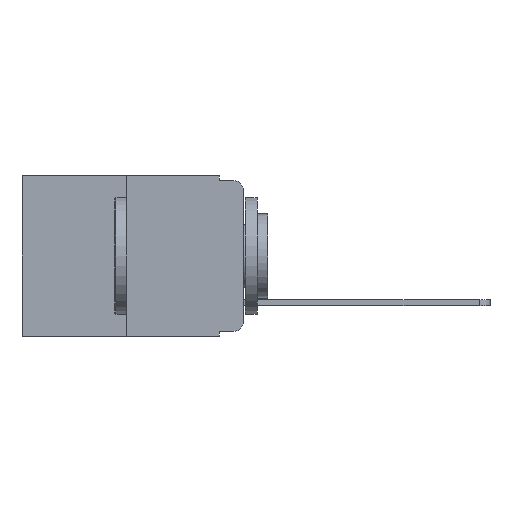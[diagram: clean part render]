
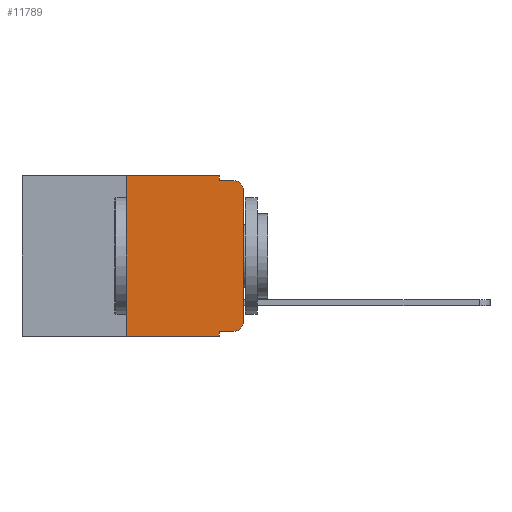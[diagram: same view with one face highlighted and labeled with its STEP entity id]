
A CAD part, left-side view. The second image highlights one B-rep face of the part: STEP entity #11789.
In plain terms, the highlighted planar face has unit normal (-1, 0, 0).
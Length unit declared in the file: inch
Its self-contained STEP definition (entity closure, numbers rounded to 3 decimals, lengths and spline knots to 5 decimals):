
#95 = EDGE_CURVE ( 'NONE', #4473, #4813, #11190, .T. ) ;
#414 = EDGE_CURVE ( 'NONE', #8009, #8805, #6182, .T. ) ;
#613 = EDGE_CURVE ( 'NONE', #2740, #1840, #8915, .T. ) ;
#783 = AXIS2_PLACEMENT_3D ( 'NONE', #10735, #5534, #11582 ) ;
#919 = CARTESIAN_POINT ( 'NONE',  ( 0., 0.051, -0.333 ) ) ;
#976 = LINE ( 'NONE', #11518, #8476 ) ;
#1075 = ORIENTED_EDGE ( 'NONE', *, *, #1500, .T. ) ;
#1089 = DIRECTION ( 'NONE',  ( 0., 0., 1. ) ) ;
#1138 = ORIENTED_EDGE ( 'NONE', *, *, #11715, .T. ) ;
#1239 = ORIENTED_EDGE ( 'NONE', *, *, #414, .F. ) ;
#1320 = ORIENTED_EDGE ( 'NONE', *, *, #1777, .F. ) ;
#1435 = ORIENTED_EDGE ( 'NONE', *, *, #3710, .F. ) ;
#1453 = CARTESIAN_POINT ( 'NONE',  ( 0., 0.02, -0.333 ) ) ;
#1490 = ORIENTED_EDGE ( 'NONE', *, *, #95, .F. ) ;
#1500 = EDGE_CURVE ( 'NONE', #1840, #4595, #9960, .T. ) ;
#1570 = ORIENTED_EDGE ( 'NONE', *, *, #6686, .T. ) ;
#1635 = ORIENTED_EDGE ( 'NONE', *, *, #5709, .F. ) ;
#1747 = CARTESIAN_POINT ( 'NONE',  ( 0., 0.25, 0. ) ) ;
#1765 = ORIENTED_EDGE ( 'NONE', *, *, #7527, .T. ) ;
#1777 = EDGE_CURVE ( 'NONE', #9561, #8009, #2238, .T. ) ;
#1840 = VERTEX_POINT ( 'NONE', #3034 ) ;
#1904 = ORIENTED_EDGE ( 'NONE', *, *, #613, .T. ) ;
#2153 = CARTESIAN_POINT ( 'NONE',  ( 0., 0.051, 0. ) ) ;
#2238 = LINE ( 'NONE', #11919, #7297 ) ;
#2255 = VECTOR ( 'NONE', #10435, 39.37008 ) ;
#2387 = DIRECTION ( 'NONE',  ( 0., 0., -1. ) ) ;
#2417 = DIRECTION ( 'NONE',  ( -1., 0., 0. ) ) ;
#2437 = CARTESIAN_POINT ( 'NONE',  ( 0., 0.02, -0.313 ) ) ;
#2740 = VERTEX_POINT ( 'NONE', #1453 ) ;
#2889 = DIRECTION ( 'NONE',  ( 0., 0., -1. ) ) ;
#3034 = CARTESIAN_POINT ( 'NONE',  ( 0., 0., -0.313 ) ) ;
#3709 = CARTESIAN_POINT ( 'NONE',  ( 0., 0.473, 0. ) ) ;
#3710 = EDGE_CURVE ( 'NONE', #4813, #9561, #11620, .T. ) ;
#4097 = CARTESIAN_POINT ( 'NONE',  ( 0., 0.25, -0.343 ) ) ;
#4186 = CARTESIAN_POINT ( 'NONE',  ( 0., 0., -0.03 ) ) ;
#4473 = VERTEX_POINT ( 'NONE', #4097 ) ;
#4595 = VERTEX_POINT ( 'NONE', #4186 ) ;
#4644 = DIRECTION ( 'NONE',  ( 0., 0., -1. ) ) ;
#4654 = CARTESIAN_POINT ( 'NONE',  ( 0., 0.051, -0.343 ) ) ;
#4674 = DIRECTION ( 'NONE',  ( 0., 0., -1. ) ) ;
#4755 = AXIS2_PLACEMENT_3D ( 'NONE', #3709, #9983, #4674 ) ;
#4813 = VERTEX_POINT ( 'NONE', #1747 ) ;
#4916 = VECTOR ( 'NONE', #8345, 39.37008 ) ;
#5203 = CARTESIAN_POINT ( 'NONE',  ( 0., 0.051, -0.01 ) ) ;
#5318 = CARTESIAN_POINT ( 'NONE',  ( 0., 0.051, -0.01 ) ) ;
#5534 = DIRECTION ( 'NONE',  ( -1., 0., 0. ) ) ;
#5709 = EDGE_CURVE ( 'NONE', #11911, #7623, #10123, .T. ) ;
#5711 = EDGE_LOOP ( 'NONE', ( #1075, #1138, #1239, #1320, #1435, #1490, #1570, #1635, #1765, #1904 ) ) ;
#5879 = CARTESIAN_POINT ( 'NONE',  ( 0., 0., 0. ) ) ;
#6182 = LINE ( 'NONE', #5203, #10528 ) ;
#6450 = CARTESIAN_POINT ( 'NONE',  ( 0., 0.051, 0. ) ) ;
#6574 = CIRCLE ( 'NONE', #783, 0.02 ) ;
#6686 = EDGE_CURVE ( 'NONE', #4473, #7623, #7024, .T. ) ;
#6853 = DIRECTION ( 'NONE',  ( 0., -1., 0. ) ) ;
#6909 = VECTOR ( 'NONE', #1089, 39.37008 ) ;
#7024 = LINE ( 'NONE', #10448, #2255 ) ;
#7231 = CARTESIAN_POINT ( 'NONE',  ( 0., 0.25, 0. ) ) ;
#7248 = DIRECTION ( 'NONE',  ( 0., -1., 0. ) ) ;
#7297 = VECTOR ( 'NONE', #4644, 39.37008 ) ;
#7420 = DIRECTION ( 'NONE',  ( 0., 0., 1. ) ) ;
#7527 = EDGE_CURVE ( 'NONE', #11911, #2740, #976, .T. ) ;
#7597 = CARTESIAN_POINT ( 'NONE',  ( 0., 0.02, -0.01 ) ) ;
#7623 = VERTEX_POINT ( 'NONE', #4654 ) ;
#7656 = AXIS2_PLACEMENT_3D ( 'NONE', #2437, #2417, #2387 ) ;
#7869 = VECTOR ( 'NONE', #2889, 39.37008 ) ;
#8009 = VERTEX_POINT ( 'NONE', #5318 ) ;
#8268 = PLANE ( 'NONE',  #4755 ) ;
#8345 = DIRECTION ( 'NONE',  ( 0., -1., 0. ) ) ;
#8476 = VECTOR ( 'NONE', #7248, 39.37008 ) ;
#8789 = CARTESIAN_POINT ( 'NONE',  ( 0., 0.473, 0. ) ) ;
#8805 = VERTEX_POINT ( 'NONE', #7597 ) ;
#8915 = CIRCLE ( 'NONE', #7656, 0.02 ) ;
#9561 = VERTEX_POINT ( 'NONE', #2153 ) ;
#9800 = FACE_OUTER_BOUND ( 'NONE', #5711, .T. ) ;
#9960 = LINE ( 'NONE', #5879, #11418 ) ;
#9983 = DIRECTION ( 'NONE',  ( 1., 0., 0. ) ) ;
#10123 = LINE ( 'NONE', #6450, #7869 ) ;
#10435 = DIRECTION ( 'NONE',  ( 0., -1., 0. ) ) ;
#10448 = CARTESIAN_POINT ( 'NONE',  ( 0., 0.473, -0.343 ) ) ;
#10528 = VECTOR ( 'NONE', #6853, 39.37008 ) ;
#10735 = CARTESIAN_POINT ( 'NONE',  ( 0., 0.02, -0.03 ) ) ;
#11190 = LINE ( 'NONE', #7231, #6909 ) ;
#11418 = VECTOR ( 'NONE', #7420, 39.37008 ) ;
#11518 = CARTESIAN_POINT ( 'NONE',  ( 0., 0.051, -0.333 ) ) ;
#11582 = DIRECTION ( 'NONE',  ( 0., 0., -1. ) ) ;
#11620 = LINE ( 'NONE', #8789, #4916 ) ;
#11715 = EDGE_CURVE ( 'NONE', #4595, #8805, #6574, .T. ) ;
#11789 = ADVANCED_FACE ( 'NONE', ( #9800 ), #8268, .F. ) ;
#11911 = VERTEX_POINT ( 'NONE', #919 ) ;
#11919 = CARTESIAN_POINT ( 'NONE',  ( 0., 0.051, 0. ) ) ;
